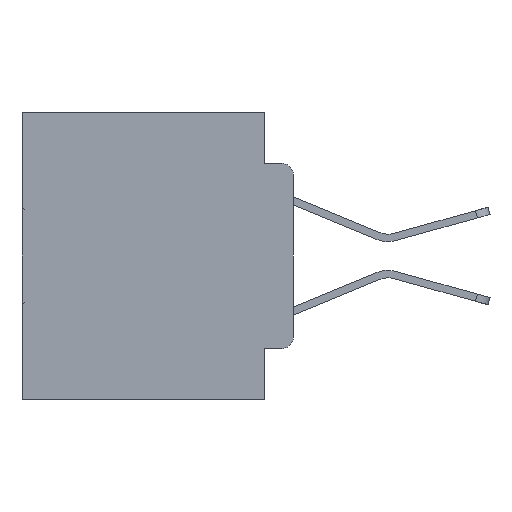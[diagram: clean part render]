
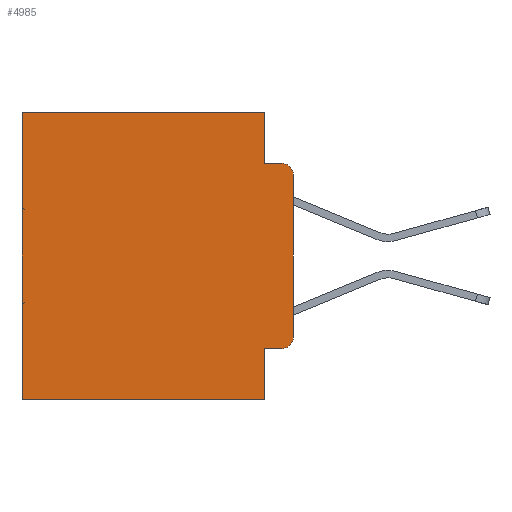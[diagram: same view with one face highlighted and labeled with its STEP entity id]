
A CAD part, left-side view. The second image highlights one B-rep face of the part: STEP entity #4985.
In plain terms, the highlighted planar face has unit normal (-1, 0, 0).
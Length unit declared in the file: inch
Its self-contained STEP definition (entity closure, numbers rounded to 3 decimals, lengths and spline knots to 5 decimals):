
#316 = DIRECTION ( 'NONE',  ( 0., -1., 0. ) ) ;
#803 = LINE ( 'NONE', #18345, #6683 ) ;
#1495 = CARTESIAN_POINT ( 'NONE',  ( 0.298, 0., 0. ) ) ;
#2756 = VERTEX_POINT ( 'NONE', #4535 ) ;
#3352 = CIRCLE ( 'NONE', #11806, 0.02 ) ;
#3415 = DIRECTION ( 'NONE',  ( 0., -1., 0. ) ) ;
#3436 = ORIENTED_EDGE ( 'NONE', *, *, #22175, .T. ) ;
#4094 = DIRECTION ( 'NONE',  ( 0., 0., -1. ) ) ;
#4493 = CARTESIAN_POINT ( 'NONE',  ( 0.298, 0.051, -0.5 ) ) ;
#4535 = CARTESIAN_POINT ( 'NONE',  ( 0.298, 0.02, -0.4115 ) ) ;
#4884 = VECTOR ( 'NONE', #27596, 39.37008 ) ;
#4985 = ADVANCED_FACE ( 'NONE', ( #11221 ), #21757, .F. ) ;
#5232 = VECTOR ( 'NONE', #316, 39.37008 ) ;
#5235 = VERTEX_POINT ( 'NONE', #11980 ) ;
#5696 = CARTESIAN_POINT ( 'NONE',  ( 0.298, 0.473, 0. ) ) ;
#6261 = DIRECTION ( 'NONE',  ( 1., 0., 0. ) ) ;
#6299 = LINE ( 'NONE', #13130, #12921 ) ;
#6397 = VECTOR ( 'NONE', #23758, 39.37008 ) ;
#6683 = VECTOR ( 'NONE', #3415, 39.37008 ) ;
#8123 = EDGE_CURVE ( 'NONE', #5235, #8292, #803, .T. ) ;
#8292 = VERTEX_POINT ( 'NONE', #31215 ) ;
#8844 = ORIENTED_EDGE ( 'NONE', *, *, #21750, .F. ) ;
#8854 = DIRECTION ( 'NONE',  ( 0., 0., -1. ) ) ;
#9802 = EDGE_CURVE ( 'NONE', #2756, #19963, #29485, .T. ) ;
#10271 = LINE ( 'NONE', #5696, #23563 ) ;
#10806 = ORIENTED_EDGE ( 'NONE', *, *, #26878, .T. ) ;
#11221 = FACE_OUTER_BOUND ( 'NONE', #13609, .T. ) ;
#11438 = VECTOR ( 'NONE', #4094, 39.37008 ) ;
#11721 = VERTEX_POINT ( 'NONE', #22486 ) ;
#11806 = AXIS2_PLACEMENT_3D ( 'NONE', #12644, #29973, #15163 ) ;
#11980 = CARTESIAN_POINT ( 'NONE',  ( 0.298, 0.051, -0.0885 ) ) ;
#12351 = CARTESIAN_POINT ( 'NONE',  ( 0.298, 0.02, -0.3915 ) ) ;
#12363 = ORIENTED_EDGE ( 'NONE', *, *, #17814, .T. ) ;
#12644 = CARTESIAN_POINT ( 'NONE',  ( 0.298, 0.02, -0.1085 ) ) ;
#12921 = VECTOR ( 'NONE', #30463, 39.37008 ) ;
#13087 = DIRECTION ( 'NONE',  ( 0., 0., -1. ) ) ;
#13130 = CARTESIAN_POINT ( 'NONE',  ( 0.298, 0., 0. ) ) ;
#13609 = EDGE_LOOP ( 'NONE', ( #28691, #10806, #27555, #8844, #12363, #3436, #26000, #26077, #14634, #15864 ) ) ;
#14092 = CARTESIAN_POINT ( 'NONE',  ( 0.298, 0., 0. ) ) ;
#14111 = VERTEX_POINT ( 'NONE', #29866 ) ;
#14598 = LINE ( 'NONE', #21239, #6397 ) ;
#14634 = ORIENTED_EDGE ( 'NONE', *, *, #16565, .T. ) ;
#14860 = DIRECTION ( 'NONE',  ( 0., 0., -1. ) ) ;
#15163 = DIRECTION ( 'NONE',  ( 0., 0., -1. ) ) ;
#15864 = ORIENTED_EDGE ( 'NONE', *, *, #9802, .T. ) ;
#15893 = EDGE_CURVE ( 'NONE', #28058, #24956, #18174, .T. ) ;
#16196 = LINE ( 'NONE', #28843, #28568 ) ;
#16241 = CARTESIAN_POINT ( 'NONE',  ( 0.298, 0., -0.3915 ) ) ;
#16565 = EDGE_CURVE ( 'NONE', #24478, #2756, #31563, .T. ) ;
#17244 = AXIS2_PLACEMENT_3D ( 'NONE', #12351, #29681, #14860 ) ;
#17814 = EDGE_CURVE ( 'NONE', #14111, #11721, #6299, .T. ) ;
#18174 = LINE ( 'NONE', #25135, #4884 ) ;
#18345 = CARTESIAN_POINT ( 'NONE',  ( 0.298, 0.051, -0.0885 ) ) ;
#19963 = VERTEX_POINT ( 'NONE', #16241 ) ;
#21239 = CARTESIAN_POINT ( 'NONE',  ( 0.298, 0.051, 0. ) ) ;
#21750 = EDGE_CURVE ( 'NONE', #14111, #5235, #16196, .T. ) ;
#21757 = PLANE ( 'NONE',  #25603 ) ;
#22175 = EDGE_CURVE ( 'NONE', #11721, #24956, #10271, .T. ) ;
#22360 = EDGE_CURVE ( 'NONE', #31613, #19963, #31203, .T. ) ;
#22486 = CARTESIAN_POINT ( 'NONE',  ( 0.298, 0.473, 0. ) ) ;
#22824 = CARTESIAN_POINT ( 'NONE',  ( 0.298, 0.051, -0.4115 ) ) ;
#23563 = VECTOR ( 'NONE', #13087, 39.37008 ) ;
#23708 = DIRECTION ( 'NONE',  ( 0., 0., -1. ) ) ;
#23758 = DIRECTION ( 'NONE',  ( 0., 0., -1. ) ) ;
#24478 = VERTEX_POINT ( 'NONE', #22824 ) ;
#24956 = VERTEX_POINT ( 'NONE', #27329 ) ;
#25135 = CARTESIAN_POINT ( 'NONE',  ( 0.298, 0., -0.5 ) ) ;
#25603 = AXIS2_PLACEMENT_3D ( 'NONE', #14092, #6261, #23708 ) ;
#26000 = ORIENTED_EDGE ( 'NONE', *, *, #15893, .F. ) ;
#26077 = ORIENTED_EDGE ( 'NONE', *, *, #27176, .F. ) ;
#26878 = EDGE_CURVE ( 'NONE', #31613, #8292, #3352, .T. ) ;
#27176 = EDGE_CURVE ( 'NONE', #24478, #28058, #14598, .T. ) ;
#27329 = CARTESIAN_POINT ( 'NONE',  ( 0.298, 0.473, -0.5 ) ) ;
#27555 = ORIENTED_EDGE ( 'NONE', *, *, #8123, .F. ) ;
#27596 = DIRECTION ( 'NONE',  ( 0., 1., 0. ) ) ;
#27771 = CARTESIAN_POINT ( 'NONE',  ( 0.298, 0., -0.1085 ) ) ;
#28058 = VERTEX_POINT ( 'NONE', #4493 ) ;
#28568 = VECTOR ( 'NONE', #8854, 39.37008 ) ;
#28691 = ORIENTED_EDGE ( 'NONE', *, *, #22360, .F. ) ;
#28843 = CARTESIAN_POINT ( 'NONE',  ( 0.298, 0.051, 0. ) ) ;
#29485 = CIRCLE ( 'NONE', #17244, 0.02 ) ;
#29681 = DIRECTION ( 'NONE',  ( -1., 0., 0. ) ) ;
#29866 = CARTESIAN_POINT ( 'NONE',  ( 0.298, 0.051, 0. ) ) ;
#29973 = DIRECTION ( 'NONE',  ( -1., 0., 0. ) ) ;
#30107 = CARTESIAN_POINT ( 'NONE',  ( 0.298, 0.051, -0.4115 ) ) ;
#30463 = DIRECTION ( 'NONE',  ( 0., 1., 0. ) ) ;
#31203 = LINE ( 'NONE', #1495, #11438 ) ;
#31215 = CARTESIAN_POINT ( 'NONE',  ( 0.298, 0.02, -0.0885 ) ) ;
#31563 = LINE ( 'NONE', #30107, #5232 ) ;
#31613 = VERTEX_POINT ( 'NONE', #27771 ) ;
